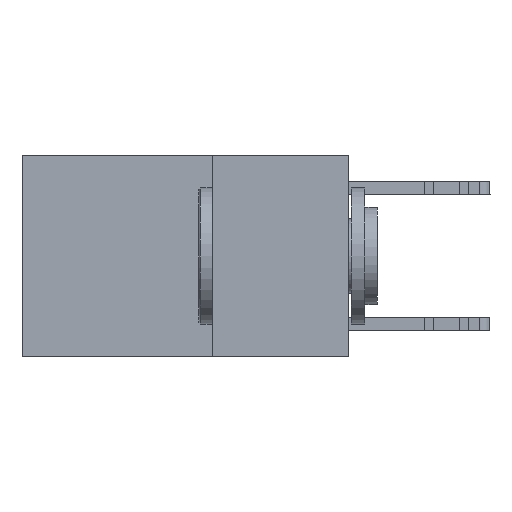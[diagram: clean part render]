
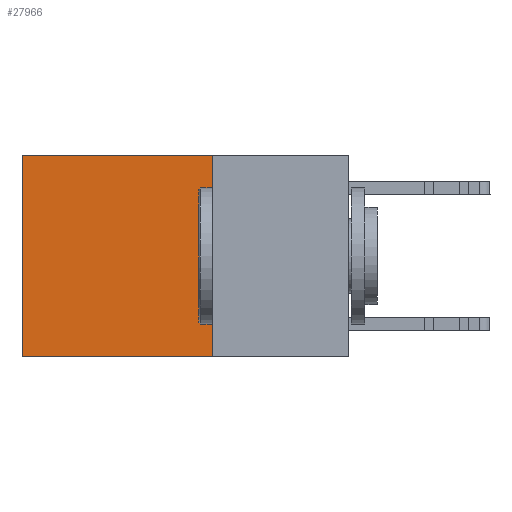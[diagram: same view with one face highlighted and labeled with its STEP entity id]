
A CAD part, left-side view. The second image highlights one B-rep face of the part: STEP entity #27966.
In plain terms, the highlighted planar face has unit normal (-1, 0, 0).
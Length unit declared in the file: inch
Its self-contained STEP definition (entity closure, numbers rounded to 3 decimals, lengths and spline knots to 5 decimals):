
#824 = CARTESIAN_POINT ( 'NONE',  ( 0.2625, 0.6, -0.37 ) ) ;
#1973 = CARTESIAN_POINT ( 'NONE',  ( 0.2625, 0.25, 0. ) ) ;
#2061 = DIRECTION ( 'NONE',  ( 1., 0., 0. ) ) ;
#2551 = ORIENTED_EDGE ( 'NONE', *, *, #8686, .F. ) ;
#3096 = CARTESIAN_POINT ( 'NONE',  ( 0.2625, 0.6, 0. ) ) ;
#3178 = CARTESIAN_POINT ( 'NONE',  ( 0.2625, 0.25, 0. ) ) ;
#4534 = AXIS2_PLACEMENT_3D ( 'NONE', #1973, #2061, #17909 ) ;
#7572 = EDGE_CURVE ( 'NONE', #8114, #10230, #19059, .T. ) ;
#7746 = VECTOR ( 'NONE', #14575, 39.37008 ) ;
#8055 = LINE ( 'NONE', #16189, #7746 ) ;
#8114 = VERTEX_POINT ( 'NONE', #3178 ) ;
#8686 = EDGE_CURVE ( 'NONE', #8114, #12607, #12680, .T. ) ;
#8882 = LINE ( 'NONE', #20145, #8936 ) ;
#8936 = VECTOR ( 'NONE', #21038, 39.37008 ) ;
#10230 = VERTEX_POINT ( 'NONE', #3096 ) ;
#10633 = ORIENTED_EDGE ( 'NONE', *, *, #25694, .T. ) ;
#11816 = EDGE_LOOP ( 'NONE', ( #10633, #22526, #2551, #24053 ) ) ;
#12569 = VECTOR ( 'NONE', #13844, 39.37008 ) ;
#12607 = VERTEX_POINT ( 'NONE', #13310 ) ;
#12680 = LINE ( 'NONE', #13460, #12569 ) ;
#13310 = CARTESIAN_POINT ( 'NONE',  ( 0.2625, 0.25, -0.37 ) ) ;
#13460 = CARTESIAN_POINT ( 'NONE',  ( 0.2625, 0.25, 0. ) ) ;
#13844 = DIRECTION ( 'NONE',  ( 0., 0., -1. ) ) ;
#14575 = DIRECTION ( 'NONE',  ( 0., 0., -1. ) ) ;
#15662 = PLANE ( 'NONE',  #4534 ) ;
#16189 = CARTESIAN_POINT ( 'NONE',  ( 0.2625, 0.6, 0. ) ) ;
#17796 = FACE_OUTER_BOUND ( 'NONE', #11816, .T. ) ;
#17909 = DIRECTION ( 'NONE',  ( 0., 0., -1. ) ) ;
#18974 = VECTOR ( 'NONE', #19950, 39.37008 ) ;
#19059 = LINE ( 'NONE', #19737, #18974 ) ;
#19737 = CARTESIAN_POINT ( 'NONE',  ( 0.2625, 0.25, 0. ) ) ;
#19950 = DIRECTION ( 'NONE',  ( 0., 1., 0. ) ) ;
#20145 = CARTESIAN_POINT ( 'NONE',  ( 0.2625, 0.25, -0.37 ) ) ;
#21038 = DIRECTION ( 'NONE',  ( 0., 1., 0. ) ) ;
#22526 = ORIENTED_EDGE ( 'NONE', *, *, #25616, .F. ) ;
#24053 = ORIENTED_EDGE ( 'NONE', *, *, #7572, .T. ) ;
#25616 = EDGE_CURVE ( 'NONE', #12607, #28294, #8882, .T. ) ;
#25694 = EDGE_CURVE ( 'NONE', #10230, #28294, #8055, .T. ) ;
#27966 = ADVANCED_FACE ( 'NONE', ( #17796 ), #15662, .F. ) ;
#28294 = VERTEX_POINT ( 'NONE', #824 ) ;
